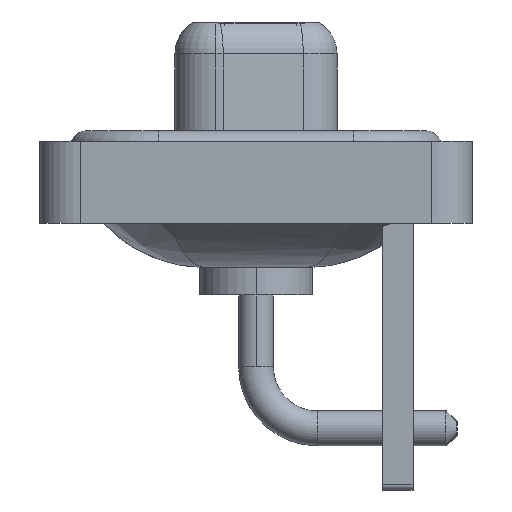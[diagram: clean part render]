
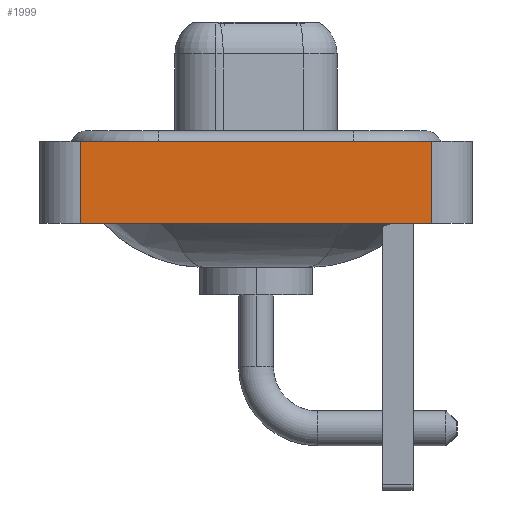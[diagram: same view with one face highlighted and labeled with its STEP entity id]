
A CAD part, left-side view. The second image highlights one B-rep face of the part: STEP entity #1999.
In plain terms, the highlighted planar face has unit normal (-1, 0, 0).
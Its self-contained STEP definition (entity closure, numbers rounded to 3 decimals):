
#442 = VECTOR ( 'NONE', #9483, 1000. ) ;
#794 = CARTESIAN_POINT ( 'NONE',  ( -7.25, -8.55, -3.6 ) ) ;
#969 = FACE_OUTER_BOUND ( 'NONE', #8974, .T. ) ;
#1835 = CARTESIAN_POINT ( 'NONE',  ( -7.25, -8.55, -3.6 ) ) ;
#1839 = CARTESIAN_POINT ( 'NONE',  ( -7.25, -8.55, 0.4 ) ) ;
#1999 = ADVANCED_FACE ( 'NONE', ( #969 ), #6464, .T. ) ;
#2923 = CARTESIAN_POINT ( 'NONE',  ( -7.25, -8.55, -3.6 ) ) ;
#3021 = LINE ( 'NONE', #1835, #3886 ) ;
#3586 = CARTESIAN_POINT ( 'NONE',  ( -7.25, -8.55, 0.4 ) ) ;
#3886 = VECTOR ( 'NONE', #17051, 1000. ) ;
#4000 = CARTESIAN_POINT ( 'NONE',  ( -7.25, -8.55, -3.6 ) ) ;
#4683 = CARTESIAN_POINT ( 'NONE',  ( -7.25, 8.55, 0.4 ) ) ;
#5864 = EDGE_CURVE ( 'NONE', #11009, #9631, #3021, .T. ) ;
#6080 = DIRECTION ( 'NONE',  ( 0., -1., 0. ) ) ;
#6233 = EDGE_CURVE ( 'NONE', #9631, #16508, #16323, .T. ) ;
#6289 = DIRECTION ( 'NONE',  ( -1., 0., 0. ) ) ;
#6464 = PLANE ( 'NONE',  #16052 ) ;
#7131 = VECTOR ( 'NONE', #6080, 1000. ) ;
#7863 = LINE ( 'NONE', #13506, #8007 ) ;
#8007 = VECTOR ( 'NONE', #14599, 1000. ) ;
#8895 = DIRECTION ( 'NONE',  ( 0., 0., 1. ) ) ;
#8974 = EDGE_LOOP ( 'NONE', ( #14204, #15918, #10465, #15095 ) ) ;
#9483 = DIRECTION ( 'NONE',  ( 0., 0., 1. ) ) ;
#9631 = VERTEX_POINT ( 'NONE', #2923 ) ;
#9931 = EDGE_CURVE ( 'NONE', #11009, #14314, #7863, .T. ) ;
#10465 = ORIENTED_EDGE ( 'NONE', *, *, #9931, .F. ) ;
#11009 = VERTEX_POINT ( 'NONE', #15983 ) ;
#11473 = LINE ( 'NONE', #1839, #7131 ) ;
#11641 = EDGE_CURVE ( 'NONE', #14314, #16508, #11473, .T. ) ;
#13506 = CARTESIAN_POINT ( 'NONE',  ( -7.25, 8.55, -3.6 ) ) ;
#14204 = ORIENTED_EDGE ( 'NONE', *, *, #6233, .T. ) ;
#14314 = VERTEX_POINT ( 'NONE', #4683 ) ;
#14599 = DIRECTION ( 'NONE',  ( 0., 0., 1. ) ) ;
#15095 = ORIENTED_EDGE ( 'NONE', *, *, #5864, .T. ) ;
#15918 = ORIENTED_EDGE ( 'NONE', *, *, #11641, .F. ) ;
#15983 = CARTESIAN_POINT ( 'NONE',  ( -7.25, 8.55, -3.6 ) ) ;
#16052 = AXIS2_PLACEMENT_3D ( 'NONE', #794, #6289, #8895 ) ;
#16323 = LINE ( 'NONE', #4000, #442 ) ;
#16508 = VERTEX_POINT ( 'NONE', #3586 ) ;
#17051 = DIRECTION ( 'NONE',  ( 0., -1., 0. ) ) ;
